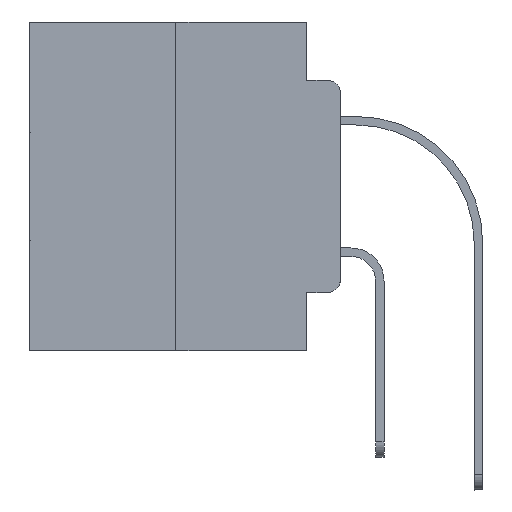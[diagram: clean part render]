
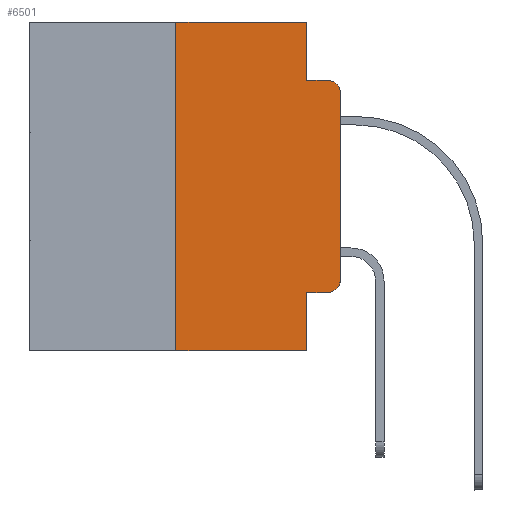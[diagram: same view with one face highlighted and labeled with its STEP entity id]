
A CAD part, left-side view. The second image highlights one B-rep face of the part: STEP entity #6501.
In plain terms, the highlighted planar face has unit normal (-1, 0, 0).
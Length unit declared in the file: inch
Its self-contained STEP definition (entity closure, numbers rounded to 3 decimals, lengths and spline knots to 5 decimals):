
#119 = ORIENTED_EDGE ( 'NONE', *, *, #13288, .F. ) ;
#159 = CARTESIAN_POINT ( 'NONE',  ( 0., 0.051, -0.4115 ) ) ;
#279 = VERTEX_POINT ( 'NONE', #1607 ) ;
#456 = DIRECTION ( 'NONE',  ( 0., 0., -1. ) ) ;
#1147 = CARTESIAN_POINT ( 'NONE',  ( 0., 0.02, -0.3915 ) ) ;
#1190 = VERTEX_POINT ( 'NONE', #11214 ) ;
#1192 = ORIENTED_EDGE ( 'NONE', *, *, #18306, .F. ) ;
#1290 = DIRECTION ( 'NONE',  ( 0., 0., 1. ) ) ;
#1607 = CARTESIAN_POINT ( 'NONE',  ( 0., 0.051, -0.0885 ) ) ;
#1621 = LINE ( 'NONE', #3799, #22227 ) ;
#2282 = DIRECTION ( 'NONE',  ( -1., 0., 0. ) ) ;
#2462 = VERTEX_POINT ( 'NONE', #11514 ) ;
#2698 = CARTESIAN_POINT ( 'NONE',  ( 0., 0.051, 0. ) ) ;
#2904 = VERTEX_POINT ( 'NONE', #16089 ) ;
#3799 = CARTESIAN_POINT ( 'NONE',  ( 0., 0., 0. ) ) ;
#3829 = EDGE_LOOP ( 'NONE', ( #5108, #25665, #18707, #18044, #119, #1192, #4573, #21716, #4744, #14890 ) ) ;
#4169 = VECTOR ( 'NONE', #29415, 39.37008 ) ;
#4189 = LINE ( 'NONE', #29712, #20800 ) ;
#4331 = CARTESIAN_POINT ( 'NONE',  ( 0., 0.25, 0. ) ) ;
#4427 = DIRECTION ( 'NONE',  ( 0., 0., -1. ) ) ;
#4573 = ORIENTED_EDGE ( 'NONE', *, *, #9800, .T. ) ;
#4744 = ORIENTED_EDGE ( 'NONE', *, *, #11877, .T. ) ;
#5108 = ORIENTED_EDGE ( 'NONE', *, *, #17893, .T. ) ;
#5166 = AXIS2_PLACEMENT_3D ( 'NONE', #14130, #2282, #4427 ) ;
#5769 = VERTEX_POINT ( 'NONE', #9969 ) ;
#6197 = LINE ( 'NONE', #23081, #27529 ) ;
#6501 = ADVANCED_FACE ( 'NONE', ( #7267 ), #28135, .F. ) ;
#6672 = CARTESIAN_POINT ( 'NONE',  ( 0., 0.25, 0. ) ) ;
#6707 = VECTOR ( 'NONE', #21096, 39.37008 ) ;
#7096 = LINE ( 'NONE', #159, #6707 ) ;
#7267 = FACE_OUTER_BOUND ( 'NONE', #3829, .T. ) ;
#8368 = CIRCLE ( 'NONE', #23567, 0.02 ) ;
#9800 = EDGE_CURVE ( 'NONE', #2462, #12939, #12701, .T. ) ;
#9969 = CARTESIAN_POINT ( 'NONE',  ( 0., 0., -0.3915 ) ) ;
#10645 = VECTOR ( 'NONE', #12089, 39.37008 ) ;
#10991 = EDGE_CURVE ( 'NONE', #279, #22648, #21759, .T. ) ;
#11214 = CARTESIAN_POINT ( 'NONE',  ( 0., 0.051, -0.4115 ) ) ;
#11408 = DIRECTION ( 'NONE',  ( 0., -1., 0. ) ) ;
#11514 = CARTESIAN_POINT ( 'NONE',  ( 0., 0.25, -0.5 ) ) ;
#11877 = EDGE_CURVE ( 'NONE', #1190, #19989, #7096, .T. ) ;
#12089 = DIRECTION ( 'NONE',  ( 0., 0., -1. ) ) ;
#12401 = EDGE_CURVE ( 'NONE', #19989, #5769, #8368, .T. ) ;
#12701 = LINE ( 'NONE', #20064, #4169 ) ;
#12726 = DIRECTION ( 'NONE',  ( 0., 0., -1. ) ) ;
#12813 = CARTESIAN_POINT ( 'NONE',  ( 0., 0.02, -0.4115 ) ) ;
#12939 = VERTEX_POINT ( 'NONE', #18942 ) ;
#13288 = EDGE_CURVE ( 'NONE', #25213, #2904, #6197, .T. ) ;
#14130 = CARTESIAN_POINT ( 'NONE',  ( 0., 0.02, -0.1085 ) ) ;
#14890 = ORIENTED_EDGE ( 'NONE', *, *, #12401, .T. ) ;
#15743 = DIRECTION ( 'NONE',  ( 0., 0., -1. ) ) ;
#16089 = CARTESIAN_POINT ( 'NONE',  ( 0., 0.051, 0. ) ) ;
#17296 = CARTESIAN_POINT ( 'NONE',  ( 0., 0.051, -0.0885 ) ) ;
#17465 = VECTOR ( 'NONE', #1290, 39.37008 ) ;
#17893 = EDGE_CURVE ( 'NONE', #5769, #26133, #1621, .T. ) ;
#18044 = ORIENTED_EDGE ( 'NONE', *, *, #21586, .F. ) ;
#18118 = CARTESIAN_POINT ( 'NONE',  ( 0., 0.02, -0.0885 ) ) ;
#18306 = EDGE_CURVE ( 'NONE', #2462, #25213, #27421, .T. ) ;
#18707 = ORIENTED_EDGE ( 'NONE', *, *, #10991, .F. ) ;
#18942 = CARTESIAN_POINT ( 'NONE',  ( 0., 0.051, -0.5 ) ) ;
#19301 = EDGE_CURVE ( 'NONE', #1190, #12939, #30376, .T. ) ;
#19919 = VECTOR ( 'NONE', #24071, 39.37008 ) ;
#19989 = VERTEX_POINT ( 'NONE', #12813 ) ;
#20064 = CARTESIAN_POINT ( 'NONE',  ( 0., 0.473, -0.5 ) ) ;
#20800 = VECTOR ( 'NONE', #12726, 39.37008 ) ;
#21096 = DIRECTION ( 'NONE',  ( 0., -1., 0. ) ) ;
#21297 = AXIS2_PLACEMENT_3D ( 'NONE', #23535, #26006, #456 ) ;
#21586 = EDGE_CURVE ( 'NONE', #2904, #279, #4189, .T. ) ;
#21716 = ORIENTED_EDGE ( 'NONE', *, *, #19301, .F. ) ;
#21759 = LINE ( 'NONE', #17296, #19919 ) ;
#22227 = VECTOR ( 'NONE', #27452, 39.37008 ) ;
#22630 = EDGE_CURVE ( 'NONE', #26133, #22648, #26288, .T. ) ;
#22648 = VERTEX_POINT ( 'NONE', #18118 ) ;
#23081 = CARTESIAN_POINT ( 'NONE',  ( 0., 0.473, 0. ) ) ;
#23535 = CARTESIAN_POINT ( 'NONE',  ( 0., 0.473, 0. ) ) ;
#23567 = AXIS2_PLACEMENT_3D ( 'NONE', #1147, #24529, #15743 ) ;
#24071 = DIRECTION ( 'NONE',  ( 0., -1., 0. ) ) ;
#24529 = DIRECTION ( 'NONE',  ( -1., 0., 0. ) ) ;
#25213 = VERTEX_POINT ( 'NONE', #4331 ) ;
#25665 = ORIENTED_EDGE ( 'NONE', *, *, #22630, .T. ) ;
#26006 = DIRECTION ( 'NONE',  ( 1., 0., 0. ) ) ;
#26133 = VERTEX_POINT ( 'NONE', #28725 ) ;
#26288 = CIRCLE ( 'NONE', #5166, 0.02 ) ;
#27421 = LINE ( 'NONE', #6672, #17465 ) ;
#27452 = DIRECTION ( 'NONE',  ( 0., 0., 1. ) ) ;
#27529 = VECTOR ( 'NONE', #11408, 39.37008 ) ;
#28135 = PLANE ( 'NONE',  #21297 ) ;
#28725 = CARTESIAN_POINT ( 'NONE',  ( 0., 0., -0.1085 ) ) ;
#29415 = DIRECTION ( 'NONE',  ( 0., -1., 0. ) ) ;
#29712 = CARTESIAN_POINT ( 'NONE',  ( 0., 0.051, 0. ) ) ;
#30376 = LINE ( 'NONE', #2698, #10645 ) ;
